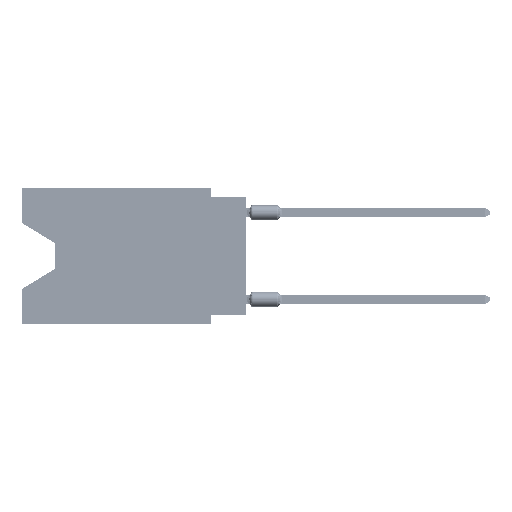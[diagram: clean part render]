
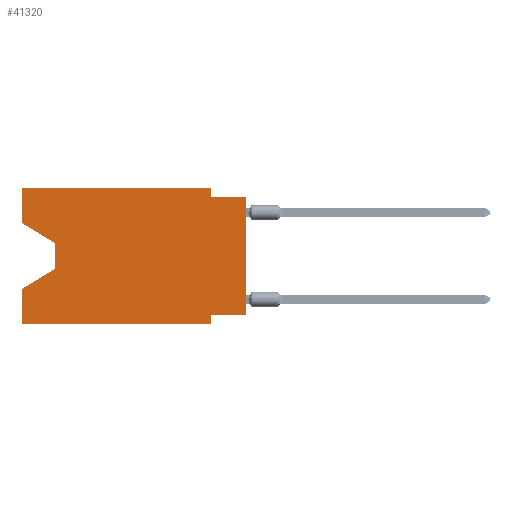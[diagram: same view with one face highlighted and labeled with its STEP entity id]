
A CAD part, left-side view. The second image highlights one B-rep face of the part: STEP entity #41320.
In plain terms, the highlighted planar face has unit normal (-1, 0, 0).
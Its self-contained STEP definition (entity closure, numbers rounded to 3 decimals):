
#291 = FACE_OUTER_BOUND ( 'NONE', #27855, .T. ) ;
#532 = EDGE_CURVE ( 'NONE', #21037, #5607, #68163, .T. ) ;
#936 = EDGE_CURVE ( 'NONE', #65765, #41821, #87345, .T. ) ;
#1935 = VECTOR ( 'NONE', #69214, 1000. ) ;
#3100 = EDGE_CURVE ( 'NONE', #41821, #18275, #69204, .T. ) ;
#3404 = CARTESIAN_POINT ( 'NONE',  ( 0., 13.97, -4.013 ) ) ;
#4609 = VERTEX_POINT ( 'NONE', #80279 ) ;
#5607 = VERTEX_POINT ( 'NONE', #41790 ) ;
#6307 = VERTEX_POINT ( 'NONE', #48311 ) ;
#6483 = VERTEX_POINT ( 'NONE', #70711 ) ;
#9459 = CARTESIAN_POINT ( 'NONE',  ( 0., 16.383, -9.906 ) ) ;
#9826 = LINE ( 'NONE', #64577, #71031 ) ;
#10814 = DIRECTION ( 'NONE',  ( 0., 0., 1. ) ) ;
#11219 = EDGE_CURVE ( 'NONE', #6307, #45194, #76792, .T. ) ;
#11607 = DIRECTION ( 'NONE',  ( 0., -1., 0. ) ) ;
#12821 = PLANE ( 'NONE',  #40323 ) ;
#12915 = CARTESIAN_POINT ( 'NONE',  ( 0., 2.54, -9.906 ) ) ;
#13806 = VECTOR ( 'NONE', #45359, 1000. ) ;
#13951 = ORIENTED_EDGE ( 'NONE', *, *, #86177, .F. ) ;
#16217 = LINE ( 'NONE', #9459, #43767 ) ;
#17546 = ORIENTED_EDGE ( 'NONE', *, *, #75541, .T. ) ;
#18275 = VERTEX_POINT ( 'NONE', #77127 ) ;
#19918 = ORIENTED_EDGE ( 'NONE', *, *, #70067, .T. ) ;
#20127 = CARTESIAN_POINT ( 'NONE',  ( 0., 16.383, -2.546 ) ) ;
#21037 = VERTEX_POINT ( 'NONE', #34492 ) ;
#22886 = ORIENTED_EDGE ( 'NONE', *, *, #532, .T. ) ;
#24257 = CARTESIAN_POINT ( 'NONE',  ( 0., 16.383, 0. ) ) ;
#24425 = EDGE_CURVE ( 'NONE', #21037, #65765, #86650, .T. ) ;
#24520 = LINE ( 'NONE', #26630, #38969 ) ;
#26630 = CARTESIAN_POINT ( 'NONE',  ( 0., 13.97, -5.893 ) ) ;
#27289 = CARTESIAN_POINT ( 'NONE',  ( 0., 16.383, 0. ) ) ;
#27855 = EDGE_LOOP ( 'NONE', ( #22886, #17546, #83364, #51507, #53520, #38257, #13951, #19918, #37041, #75568, #81908, #53257 ) ) ;
#29279 = VECTOR ( 'NONE', #42149, 1000. ) ;
#29667 = VECTOR ( 'NONE', #87448, 1000. ) ;
#30143 = CARTESIAN_POINT ( 'NONE',  ( 0., 2.54, 0. ) ) ;
#31420 = DIRECTION ( 'NONE',  ( 0., -1., 0. ) ) ;
#33051 = CARTESIAN_POINT ( 'NONE',  ( 0., 16.383, 0. ) ) ;
#33765 = CARTESIAN_POINT ( 'NONE',  ( 0., 13.97, -5.893 ) ) ;
#33833 = EDGE_CURVE ( 'NONE', #53536, #4609, #24520, .T. ) ;
#34492 = CARTESIAN_POINT ( 'NONE',  ( 0., 16.383, -2.546 ) ) ;
#34812 = DIRECTION ( 'NONE',  ( 1., 0., 0. ) ) ;
#35342 = CARTESIAN_POINT ( 'NONE',  ( 0., 16.383, -9.906 ) ) ;
#35500 = VECTOR ( 'NONE', #54386, 1000. ) ;
#36876 = VECTOR ( 'NONE', #63554, 1000. ) ;
#37041 = ORIENTED_EDGE ( 'NONE', *, *, #50169, .F. ) ;
#38257 = ORIENTED_EDGE ( 'NONE', *, *, #11219, .F. ) ;
#38969 = VECTOR ( 'NONE', #79276, 1000. ) ;
#39355 = DIRECTION ( 'NONE',  ( 0., -1., 0. ) ) ;
#40185 = DIRECTION ( 'NONE',  ( 0., 0., -1. ) ) ;
#40323 = AXIS2_PLACEMENT_3D ( 'NONE', #82805, #34812, #40185 ) ;
#41251 = LINE ( 'NONE', #61927, #29279 ) ;
#41320 = ADVANCED_FACE ( 'NONE', ( #291 ), #12821, .F. ) ;
#41790 = CARTESIAN_POINT ( 'NONE',  ( 0., 13.97, -4.013 ) ) ;
#41821 = VERTEX_POINT ( 'NONE', #30143 ) ;
#42149 = DIRECTION ( 'NONE',  ( 0., 0., 1. ) ) ;
#43128 = CARTESIAN_POINT ( 'NONE',  ( 0., 2.54, -9.906 ) ) ;
#43767 = VECTOR ( 'NONE', #31420, 1000. ) ;
#45111 = CARTESIAN_POINT ( 'NONE',  ( 0., 0., -9.271 ) ) ;
#45194 = VERTEX_POINT ( 'NONE', #12915 ) ;
#45243 = EDGE_CURVE ( 'NONE', #50370, #4609, #85745, .T. ) ;
#45359 = DIRECTION ( 'NONE',  ( 0., 0., 1. ) ) ;
#48311 = CARTESIAN_POINT ( 'NONE',  ( 0., 2.54, -9.271 ) ) ;
#50169 = EDGE_CURVE ( 'NONE', #18275, #6483, #9826, .T. ) ;
#50370 = VERTEX_POINT ( 'NONE', #35342 ) ;
#51507 = ORIENTED_EDGE ( 'NONE', *, *, #45243, .F. ) ;
#53257 = ORIENTED_EDGE ( 'NONE', *, *, #24425, .F. ) ;
#53520 = ORIENTED_EDGE ( 'NONE', *, *, #66204, .T. ) ;
#53536 = VERTEX_POINT ( 'NONE', #33765 ) ;
#54386 = DIRECTION ( 'NONE',  ( 0., 0., -1. ) ) ;
#59847 = VECTOR ( 'NONE', #39355, 1000. ) ;
#61927 = CARTESIAN_POINT ( 'NONE',  ( 0., 0., 0. ) ) ;
#62883 = CARTESIAN_POINT ( 'NONE',  ( 0., 2.54, 0. ) ) ;
#63554 = DIRECTION ( 'NONE',  ( 0., 0., -1. ) ) ;
#64577 = CARTESIAN_POINT ( 'NONE',  ( 0., 0., -0.635 ) ) ;
#64882 = LINE ( 'NONE', #3404, #36876 ) ;
#65765 = VERTEX_POINT ( 'NONE', #70736 ) ;
#66204 = EDGE_CURVE ( 'NONE', #50370, #45194, #16217, .T. ) ;
#68163 = LINE ( 'NONE', #20127, #29667 ) ;
#69204 = LINE ( 'NONE', #62883, #35500 ) ;
#69214 = DIRECTION ( 'NONE',  ( 0., 0., -1. ) ) ;
#70067 = EDGE_CURVE ( 'NONE', #79498, #6483, #41251, .T. ) ;
#70711 = CARTESIAN_POINT ( 'NONE',  ( 0., 0., -0.635 ) ) ;
#70736 = CARTESIAN_POINT ( 'NONE',  ( 0., 16.383, 0. ) ) ;
#71031 = VECTOR ( 'NONE', #11607, 1000. ) ;
#75541 = EDGE_CURVE ( 'NONE', #5607, #53536, #64882, .T. ) ;
#75568 = ORIENTED_EDGE ( 'NONE', *, *, #3100, .F. ) ;
#76792 = LINE ( 'NONE', #43128, #1935 ) ;
#77127 = CARTESIAN_POINT ( 'NONE',  ( 0., 2.54, -0.635 ) ) ;
#78411 = DIRECTION ( 'NONE',  ( 0., 1., 0. ) ) ;
#78594 = VECTOR ( 'NONE', #78411, 1000. ) ;
#79276 = DIRECTION ( 'NONE',  ( 0., 0.855, -0.519 ) ) ;
#79498 = VERTEX_POINT ( 'NONE', #45111 ) ;
#80279 = CARTESIAN_POINT ( 'NONE',  ( 0., 16.383, -7.36 ) ) ;
#81874 = VECTOR ( 'NONE', #10814, 1000. ) ;
#81908 = ORIENTED_EDGE ( 'NONE', *, *, #936, .F. ) ;
#82805 = CARTESIAN_POINT ( 'NONE',  ( 0., 16.383, 0. ) ) ;
#83364 = ORIENTED_EDGE ( 'NONE', *, *, #33833, .T. ) ;
#85158 = CARTESIAN_POINT ( 'NONE',  ( 0., 0., -9.271 ) ) ;
#85591 = LINE ( 'NONE', #85158, #78594 ) ;
#85745 = LINE ( 'NONE', #24257, #81874 ) ;
#86177 = EDGE_CURVE ( 'NONE', #79498, #6307, #85591, .T. ) ;
#86650 = LINE ( 'NONE', #27289, #13806 ) ;
#87345 = LINE ( 'NONE', #33051, #59847 ) ;
#87448 = DIRECTION ( 'NONE',  ( 0., -0.855, -0.519 ) ) ;
